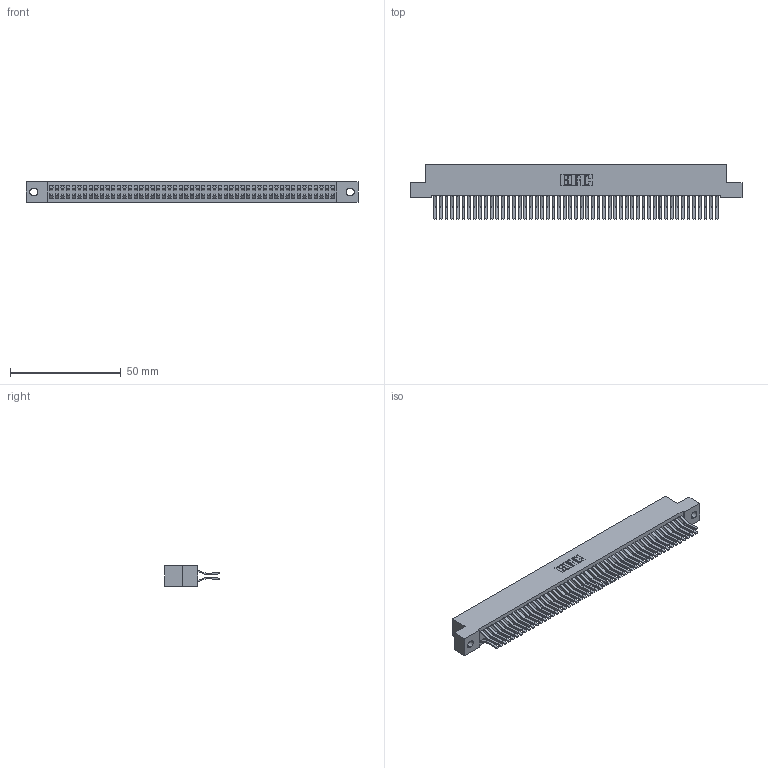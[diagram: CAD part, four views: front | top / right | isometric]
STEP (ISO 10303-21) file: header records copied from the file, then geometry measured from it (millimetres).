
FILE_DESCRIPTION (( 'STEP AP203' ), '1' );
FILE_NAME ('342-102-560-202.STEP', '2018-08-14T05:45:42', ( '' ), ( '' ), 'SwSTEP 2.0', 'SolidWorks 2016', '' );
FILE_SCHEMA (( 'CONFIG_CONTROL_DESIGN' ));
Length unit declared in the file: inch
Products named in the file (3): 342 Part_.128 Slot; 345-292-001_560 Tail; 342-102-560-202
Assembly tree (103 placements, depth 2):
  342-102-560-202
    342 Part_.128 Slot
    345-292-001_560 Tail  x102
Bounding box: 149.86 x 24.78 x 9.4 mm (x, y, z)
Volume: 14125 mm3; surface area: 24579 mm2
Topology: 103 solids, 103 shells, 5622 faces, 16733 edges, 11018 vertices
Faces by surface type: plane 3742, cylinder 1880
Entity records: 31737 total; most frequent: CARTESIAN_POINT 5250, ORIENTED_EDGE 5186, DIRECTION 4473, EDGE_CURVE 2593, LINE 2461, VECTOR 2461, VERTEX_POINT 1726, AXIS2_PLACEMENT_3D 1006
